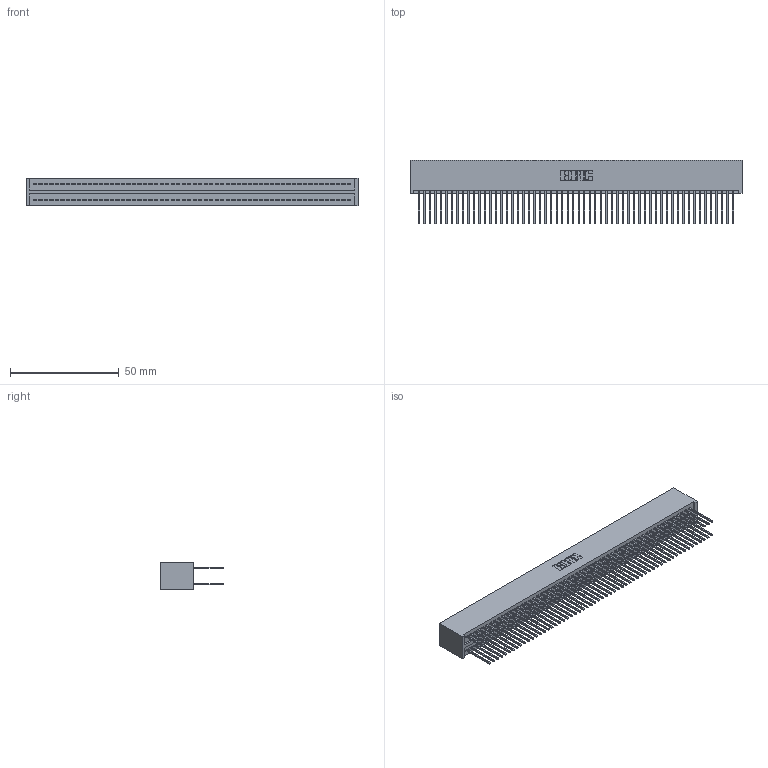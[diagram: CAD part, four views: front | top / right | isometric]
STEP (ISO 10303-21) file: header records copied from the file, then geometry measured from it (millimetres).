
FILE_DESCRIPTION (( 'STEP AP203' ), '1' );
FILE_NAME ('325-116-540-201.STEP', '2020-02-25T08:20:25', ( '' ), ( '' ), 'SwSTEP 2.0', 'SolidWorks 2016', '' );
FILE_SCHEMA (( 'CONFIG_CONTROL_DESIGN' ));
Length unit declared in the file: inch
Products named in the file (3): 325 Part_Lugless; 325-116-540-201; 325-292-001_325-293-140
Assembly tree (117 placements, depth 2):
  325-116-540-201
    325 Part_Lugless
    325-292-001_325-293-140  x116
Bounding box: 152.96 x 29.46 x 12.45 mm (x, y, z)
Volume: 20936.1 mm3; surface area: 28474 mm2
Topology: 117 solids, 117 shells, 6138 faces, 18267 edges, 12022 vertices
Faces by surface type: plane 4242, cylinder 1896
Entity records: 34985 total; most frequent: CARTESIAN_POINT 5778, ORIENTED_EDGE 5714, DIRECTION 4901, EDGE_CURVE 2857, VECTOR 2737, LINE 2737, VERTEX_POINT 1902, AXIS2_PLACEMENT_3D 1082
